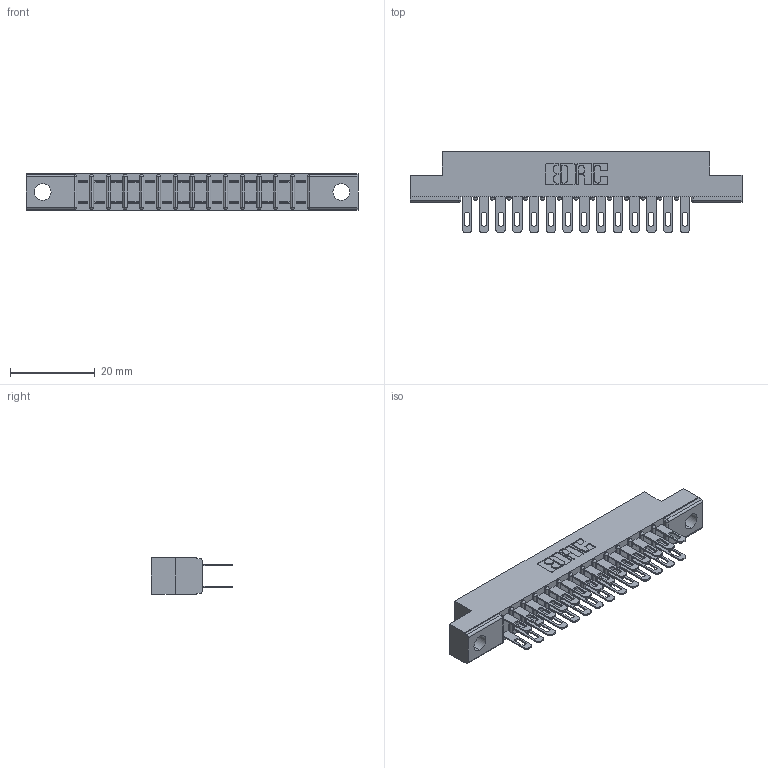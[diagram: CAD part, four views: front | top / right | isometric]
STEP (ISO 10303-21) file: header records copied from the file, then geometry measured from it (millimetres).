
FILE_DESCRIPTION (( 'STEP AP203' ), '1' );
FILE_NAME ('307-028-400-202.STEP', '2020-09-29T07:21:47', ( '' ), ( '' ), 'SwSTEP 2.0', 'SolidWorks 2020', '' );
FILE_SCHEMA (( 'CONFIG_CONTROL_DESIGN' ));
Length unit declared in the file: inch
Products named in the file (3): 307-028-400-202; 307-290-001_500; 307 Part_.128 Dia Mounting Holes
Assembly tree (29 placements, depth 2):
  307-028-400-202
    307 Part_.128 Dia Mounting Holes
    307-290-001_500  x28
Bounding box: 78.49 x 19.18 x 8.71 mm (x, y, z)
Volume: 5127.1 mm3; surface area: 8930.4 mm2
Topology: 29 solids, 29 shells, 1421 faces, 3963 edges, 2562 vertices
Faces by surface type: plane 910, cylinder 481, sphere 30
Entity records: 15878 total; most frequent: CARTESIAN_POINT 2602, ORIENTED_EDGE 2574, DIRECTION 2563, EDGE_CURVE 1287, VECTOR 973, LINE 973, VERTEX_POINT 834, AXIS2_PLACEMENT_3D 795
